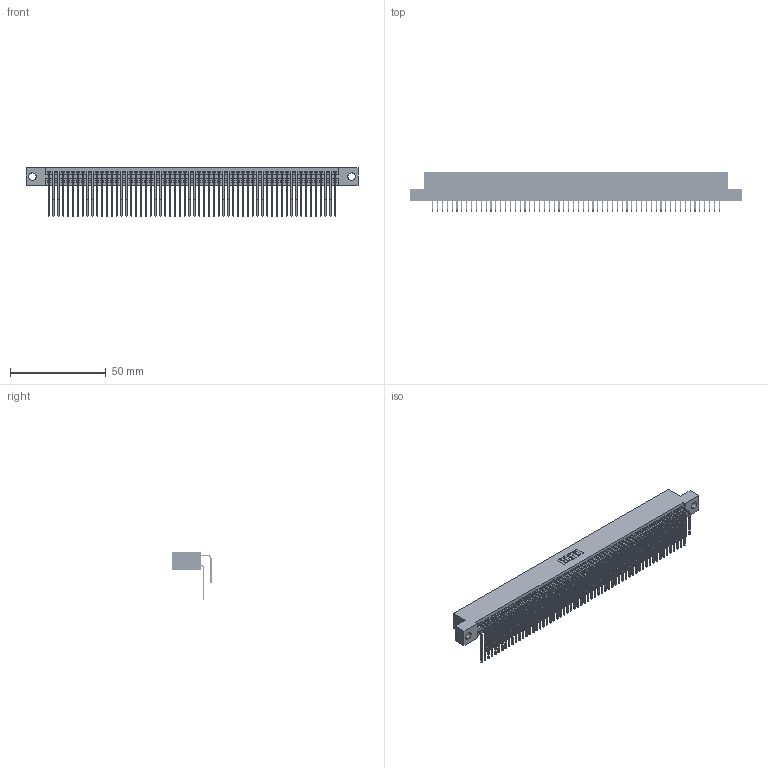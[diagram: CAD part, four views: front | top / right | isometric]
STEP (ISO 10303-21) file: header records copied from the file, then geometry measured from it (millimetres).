
FILE_DESCRIPTION (( 'STEP AP203' ), '1' );
FILE_NAME ('395-120-559-204.STEP', '2021-06-17T21:05:48', ( '' ), ( '' ), 'SwSTEP 2.0', 'SolidWorks 2020', '' );
FILE_SCHEMA (( 'CONFIG_CONTROL_DESIGN' ));
Length unit declared in the file: inch
Products named in the file (4): 345-292-001_558 559 Tail - 1; 395-120-559-204; 345-292-001_559 Tail - 2; 345 Part_Flush Mounting Lugs - 0.156 Dia-TI
Assembly tree (121 placements, depth 2):
  395-120-559-204
    345 Part_Flush Mounting Lugs - 0.156 Dia-TI
    345-292-001_558 559 Tail - 1  x60
    345-292-001_559 Tail - 2  x60
Bounding box: 173.61 x 20.56 x 25.53 mm (x, y, z)
Volume: 17617.9 mm3; surface area: 29497.7 mm2
Topology: 121 solids, 121 shells, 6380 faces, 18977 edges, 12490 vertices
Faces by surface type: plane 4294, cylinder 2086
Entity records: 46725 total; most frequent: CARTESIAN_POINT 7865, ORIENTED_EDGE 7746, DIRECTION 6885, EDGE_CURVE 3873, VECTOR 3461, LINE 3461, VERTEX_POINT 2578, AXIS2_PLACEMENT_3D 1712
